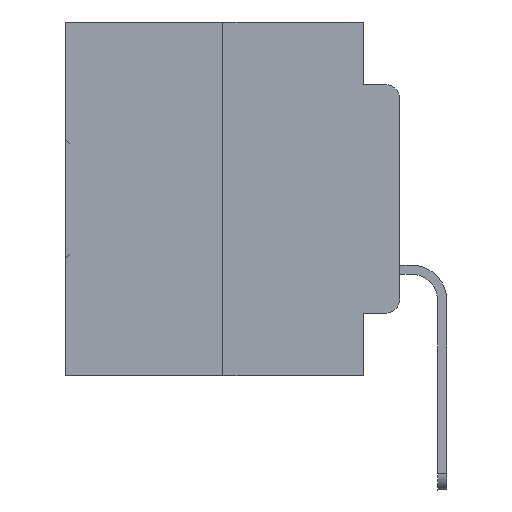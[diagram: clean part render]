
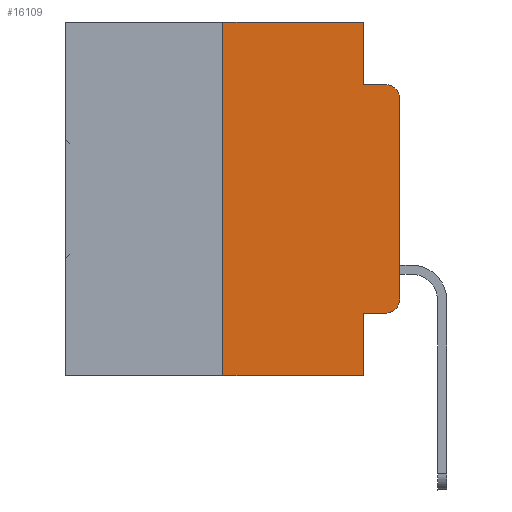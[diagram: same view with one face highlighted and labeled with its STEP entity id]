
A CAD part, left-side view. The second image highlights one B-rep face of the part: STEP entity #16109.
In plain terms, the highlighted planar face has unit normal (-1, 0, 0).
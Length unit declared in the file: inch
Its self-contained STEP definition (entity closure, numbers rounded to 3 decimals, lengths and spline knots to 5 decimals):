
#75 = AXIS2_PLACEMENT_3D ( 'NONE', #26098, #10830, #8653 ) ;
#76 = DIRECTION ( 'NONE',  ( 0., 0., -1. ) ) ;
#249 = CARTESIAN_POINT ( 'NONE',  ( 0., 0.02, -0.0885 ) ) ;
#2008 = CARTESIAN_POINT ( 'NONE',  ( 0., 0.473, 0. ) ) ;
#2323 = EDGE_LOOP ( 'NONE', ( #13889, #5724, #20123, #32719, #6606, #16572, #25250, #22697, #22028, #13036 ) ) ;
#2344 = DIRECTION ( 'NONE',  ( 1., 0., 0. ) ) ;
#2836 = LINE ( 'NONE', #23629, #12311 ) ;
#3102 = LINE ( 'NONE', #25888, #22485 ) ;
#3356 = CARTESIAN_POINT ( 'NONE',  ( 0., 0., -0.1085 ) ) ;
#4307 = CARTESIAN_POINT ( 'NONE',  ( 0., 0.051, -0.5 ) ) ;
#4309 = VERTEX_POINT ( 'NONE', #7152 ) ;
#5136 = VECTOR ( 'NONE', #14897, 39.37008 ) ;
#5724 = ORIENTED_EDGE ( 'NONE', *, *, #20108, .T. ) ;
#6052 = VECTOR ( 'NONE', #27158, 39.37008 ) ;
#6433 = AXIS2_PLACEMENT_3D ( 'NONE', #28791, #21005, #31130 ) ;
#6606 = ORIENTED_EDGE ( 'NONE', *, *, #14188, .F. ) ;
#7080 = DIRECTION ( 'NONE',  ( 0., 0., 1. ) ) ;
#7152 = CARTESIAN_POINT ( 'NONE',  ( 0., 0.25, -0.5 ) ) ;
#7249 = CARTESIAN_POINT ( 'NONE',  ( 0., 0.25, 0. ) ) ;
#7378 = LINE ( 'NONE', #9380, #22963 ) ;
#7704 = VECTOR ( 'NONE', #76, 39.37008 ) ;
#8324 = DIRECTION ( 'NONE',  ( 0., -1., 0. ) ) ;
#8357 = CARTESIAN_POINT ( 'NONE',  ( 0., 0.051, -0.0885 ) ) ;
#8653 = DIRECTION ( 'NONE',  ( 0., 0., -1. ) ) ;
#8727 = VERTEX_POINT ( 'NONE', #4307 ) ;
#8999 = EDGE_CURVE ( 'NONE', #22543, #18133, #9409, .T. ) ;
#9089 = CARTESIAN_POINT ( 'NONE',  ( 0., 0., 0. ) ) ;
#9380 = CARTESIAN_POINT ( 'NONE',  ( 0., 0.473, -0.5 ) ) ;
#9409 = LINE ( 'NONE', #9089, #15091 ) ;
#10830 = DIRECTION ( 'NONE',  ( -1., 0., 0. ) ) ;
#12023 = DIRECTION ( 'NONE',  ( 0., 0., -1. ) ) ;
#12311 = VECTOR ( 'NONE', #8324, 39.37008 ) ;
#13036 = ORIENTED_EDGE ( 'NONE', *, *, #30553, .T. ) ;
#13829 = VERTEX_POINT ( 'NONE', #24223 ) ;
#13874 = CIRCLE ( 'NONE', #6433, 0.02 ) ;
#13889 = ORIENTED_EDGE ( 'NONE', *, *, #8999, .T. ) ;
#14188 = EDGE_CURVE ( 'NONE', #25579, #18717, #26339, .T. ) ;
#14658 = CARTESIAN_POINT ( 'NONE',  ( 0., 0., -0.3915 ) ) ;
#14888 = LINE ( 'NONE', #22862, #7704 ) ;
#14897 = DIRECTION ( 'NONE',  ( 0., 0., 1. ) ) ;
#14940 = EDGE_CURVE ( 'NONE', #18323, #13829, #3102, .T. ) ;
#15091 = VECTOR ( 'NONE', #7080, 39.37008 ) ;
#15170 = FACE_OUTER_BOUND ( 'NONE', #2323, .T. ) ;
#15798 = VERTEX_POINT ( 'NONE', #8357 ) ;
#15878 = CARTESIAN_POINT ( 'NONE',  ( 0., 0.473, 0. ) ) ;
#16109 = ADVANCED_FACE ( 'NONE', ( #15170 ), #24798, .F. ) ;
#16572 = ORIENTED_EDGE ( 'NONE', *, *, #24685, .F. ) ;
#18133 = VERTEX_POINT ( 'NONE', #3356 ) ;
#18323 = VERTEX_POINT ( 'NONE', #24454 ) ;
#18516 = DIRECTION ( 'NONE',  ( 0., -1., 0. ) ) ;
#18717 = VERTEX_POINT ( 'NONE', #23934 ) ;
#20108 = EDGE_CURVE ( 'NONE', #18133, #26894, #13874, .T. ) ;
#20123 = ORIENTED_EDGE ( 'NONE', *, *, #30480, .F. ) ;
#21005 = DIRECTION ( 'NONE',  ( -1., 0., 0. ) ) ;
#21063 = EDGE_CURVE ( 'NONE', #4309, #8727, #7378, .T. ) ;
#21333 = CIRCLE ( 'NONE', #75, 0.02 ) ;
#21864 = DIRECTION ( 'NONE',  ( 0., -1., 0. ) ) ;
#22028 = ORIENTED_EDGE ( 'NONE', *, *, #14940, .T. ) ;
#22383 = LINE ( 'NONE', #7249, #5136 ) ;
#22433 = VECTOR ( 'NONE', #18516, 39.37008 ) ;
#22485 = VECTOR ( 'NONE', #28869, 39.37008 ) ;
#22543 = VERTEX_POINT ( 'NONE', #14658 ) ;
#22697 = ORIENTED_EDGE ( 'NONE', *, *, #22897, .F. ) ;
#22862 = CARTESIAN_POINT ( 'NONE',  ( 0., 0.051, 0. ) ) ;
#22897 = EDGE_CURVE ( 'NONE', #18323, #8727, #14888, .T. ) ;
#22963 = VECTOR ( 'NONE', #21864, 39.37008 ) ;
#23629 = CARTESIAN_POINT ( 'NONE',  ( 0., 0.051, -0.0885 ) ) ;
#23934 = CARTESIAN_POINT ( 'NONE',  ( 0., 0.051, 0. ) ) ;
#24142 = AXIS2_PLACEMENT_3D ( 'NONE', #2008, #2344, #12023 ) ;
#24223 = CARTESIAN_POINT ( 'NONE',  ( 0., 0.02, -0.4115 ) ) ;
#24454 = CARTESIAN_POINT ( 'NONE',  ( 0., 0.051, -0.4115 ) ) ;
#24685 = EDGE_CURVE ( 'NONE', #4309, #25579, #22383, .T. ) ;
#24798 = PLANE ( 'NONE',  #24142 ) ;
#25194 = CARTESIAN_POINT ( 'NONE',  ( 0., 0.25, 0. ) ) ;
#25250 = ORIENTED_EDGE ( 'NONE', *, *, #21063, .T. ) ;
#25579 = VERTEX_POINT ( 'NONE', #25194 ) ;
#25888 = CARTESIAN_POINT ( 'NONE',  ( 0., 0.051, -0.4115 ) ) ;
#26098 = CARTESIAN_POINT ( 'NONE',  ( 0., 0.02, -0.3915 ) ) ;
#26339 = LINE ( 'NONE', #15878, #22433 ) ;
#26894 = VERTEX_POINT ( 'NONE', #249 ) ;
#27158 = DIRECTION ( 'NONE',  ( 0., 0., -1. ) ) ;
#27841 = CARTESIAN_POINT ( 'NONE',  ( 0., 0.051, 0. ) ) ;
#28791 = CARTESIAN_POINT ( 'NONE',  ( 0., 0.02, -0.1085 ) ) ;
#28869 = DIRECTION ( 'NONE',  ( 0., -1., 0. ) ) ;
#30151 = LINE ( 'NONE', #27841, #6052 ) ;
#30480 = EDGE_CURVE ( 'NONE', #15798, #26894, #2836, .T. ) ;
#30553 = EDGE_CURVE ( 'NONE', #13829, #22543, #21333, .T. ) ;
#31130 = DIRECTION ( 'NONE',  ( 0., 0., -1. ) ) ;
#32686 = EDGE_CURVE ( 'NONE', #18717, #15798, #30151, .T. ) ;
#32719 = ORIENTED_EDGE ( 'NONE', *, *, #32686, .F. ) ;
